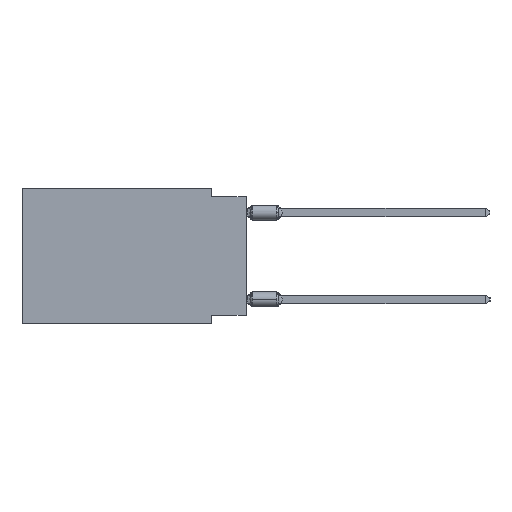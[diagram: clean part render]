
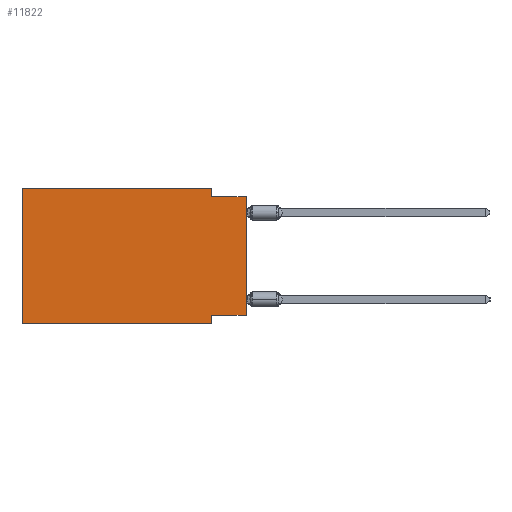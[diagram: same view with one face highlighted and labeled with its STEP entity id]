
A CAD part, left-side view. The second image highlights one B-rep face of the part: STEP entity #11822.
In plain terms, the highlighted planar face has unit normal (-1, 0, 0).
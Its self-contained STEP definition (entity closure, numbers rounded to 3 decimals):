
#471 = ORIENTED_EDGE ( 'NONE', *, *, #29640, .T. ) ;
#574 = DIRECTION ( 'NONE',  ( 0., 0., 1. ) ) ;
#1359 = CARTESIAN_POINT ( 'NONE',  ( 0., 2.54, -9.271 ) ) ;
#1633 = CARTESIAN_POINT ( 'NONE',  ( 0., 16.383, 0. ) ) ;
#1835 = PLANE ( 'NONE',  #9111 ) ;
#3413 = CARTESIAN_POINT ( 'NONE',  ( 0., 16.383, 0. ) ) ;
#3858 = DIRECTION ( 'NONE',  ( 0., 1., 0. ) ) ;
#5912 = CARTESIAN_POINT ( 'NONE',  ( 0., 0., -0.635 ) ) ;
#6122 = DIRECTION ( 'NONE',  ( 0., -1., 0. ) ) ;
#7044 = LINE ( 'NONE', #39403, #34932 ) ;
#7478 = VECTOR ( 'NONE', #3858, 1000. ) ;
#8260 = CARTESIAN_POINT ( 'NONE',  ( 0., 2.54, -9.906 ) ) ;
#9111 = AXIS2_PLACEMENT_3D ( 'NONE', #1633, #24035, #32763 ) ;
#9975 = ORIENTED_EDGE ( 'NONE', *, *, #31829, .F. ) ;
#10569 = DIRECTION ( 'NONE',  ( 0., 0., -1. ) ) ;
#11250 = EDGE_CURVE ( 'NONE', #37396, #24727, #7044, .T. ) ;
#11586 = FACE_OUTER_BOUND ( 'NONE', #11885, .T. ) ;
#11737 = DIRECTION ( 'NONE',  ( 0., 0., 1. ) ) ;
#11756 = EDGE_CURVE ( 'NONE', #24727, #28451, #19258, .T. ) ;
#11822 = ADVANCED_FACE ( 'NONE', ( #11586 ), #1835, .F. ) ;
#11885 = EDGE_LOOP ( 'NONE', ( #35892, #33816, #36733, #9975, #25058, #471, #22476, #16232 ) ) ;
#12989 = VERTEX_POINT ( 'NONE', #32152 ) ;
#13712 = EDGE_CURVE ( 'NONE', #38329, #28451, #21879, .T. ) ;
#14573 = EDGE_CURVE ( 'NONE', #18882, #12989, #29222, .T. ) ;
#14579 = VECTOR ( 'NONE', #574, 1000. ) ;
#14955 = VERTEX_POINT ( 'NONE', #19602 ) ;
#16232 = ORIENTED_EDGE ( 'NONE', *, *, #19839, .F. ) ;
#17740 = VECTOR ( 'NONE', #34944, 1000. ) ;
#18767 = CARTESIAN_POINT ( 'NONE',  ( 0., 0., 0. ) ) ;
#18882 = VERTEX_POINT ( 'NONE', #28877 ) ;
#19258 = LINE ( 'NONE', #29456, #21710 ) ;
#19602 = CARTESIAN_POINT ( 'NONE',  ( 0., 2.54, -9.906 ) ) ;
#19610 = CARTESIAN_POINT ( 'NONE',  ( 0., 0., -9.271 ) ) ;
#19839 = EDGE_CURVE ( 'NONE', #38329, #39117, #29587, .T. ) ;
#21710 = VECTOR ( 'NONE', #23015, 1000. ) ;
#21879 = LINE ( 'NONE', #18767, #30447 ) ;
#22476 = ORIENTED_EDGE ( 'NONE', *, *, #40483, .F. ) ;
#23015 = DIRECTION ( 'NONE',  ( 0., -1., 0. ) ) ;
#23023 = VECTOR ( 'NONE', #6122, 1000. ) ;
#23190 = CARTESIAN_POINT ( 'NONE',  ( 0., 16.383, 0. ) ) ;
#23832 = LINE ( 'NONE', #8260, #37186 ) ;
#24035 = DIRECTION ( 'NONE',  ( 1., 0., 0. ) ) ;
#24727 = VERTEX_POINT ( 'NONE', #35439 ) ;
#24917 = CARTESIAN_POINT ( 'NONE',  ( 0., 2.54, 0. ) ) ;
#25058 = ORIENTED_EDGE ( 'NONE', *, *, #14573, .F. ) ;
#25439 = CARTESIAN_POINT ( 'NONE',  ( 0., 16.383, -9.906 ) ) ;
#28451 = VERTEX_POINT ( 'NONE', #5912 ) ;
#28877 = CARTESIAN_POINT ( 'NONE',  ( 0., 16.383, -9.906 ) ) ;
#29222 = LINE ( 'NONE', #23190, #14579 ) ;
#29456 = CARTESIAN_POINT ( 'NONE',  ( 0., 0., -0.635 ) ) ;
#29587 = LINE ( 'NONE', #19610, #7478 ) ;
#29640 = EDGE_CURVE ( 'NONE', #18882, #14955, #38497, .T. ) ;
#30447 = VECTOR ( 'NONE', #11737, 1000. ) ;
#31829 = EDGE_CURVE ( 'NONE', #12989, #37396, #37838, .T. ) ;
#32152 = CARTESIAN_POINT ( 'NONE',  ( 0., 16.383, 0. ) ) ;
#32763 = DIRECTION ( 'NONE',  ( 0., 0., -1. ) ) ;
#33816 = ORIENTED_EDGE ( 'NONE', *, *, #11756, .F. ) ;
#34932 = VECTOR ( 'NONE', #10569, 1000. ) ;
#34944 = DIRECTION ( 'NONE',  ( 0., -1., 0. ) ) ;
#35439 = CARTESIAN_POINT ( 'NONE',  ( 0., 2.54, -0.635 ) ) ;
#35892 = ORIENTED_EDGE ( 'NONE', *, *, #13712, .T. ) ;
#36733 = ORIENTED_EDGE ( 'NONE', *, *, #11250, .F. ) ;
#37186 = VECTOR ( 'NONE', #40393, 1000. ) ;
#37396 = VERTEX_POINT ( 'NONE', #24917 ) ;
#37838 = LINE ( 'NONE', #3413, #17740 ) ;
#38234 = CARTESIAN_POINT ( 'NONE',  ( 0., 0., -9.271 ) ) ;
#38329 = VERTEX_POINT ( 'NONE', #38234 ) ;
#38497 = LINE ( 'NONE', #25439, #23023 ) ;
#39117 = VERTEX_POINT ( 'NONE', #1359 ) ;
#39403 = CARTESIAN_POINT ( 'NONE',  ( 0., 2.54, 0. ) ) ;
#40393 = DIRECTION ( 'NONE',  ( 0., 0., -1. ) ) ;
#40483 = EDGE_CURVE ( 'NONE', #39117, #14955, #23832, .T. ) ;
